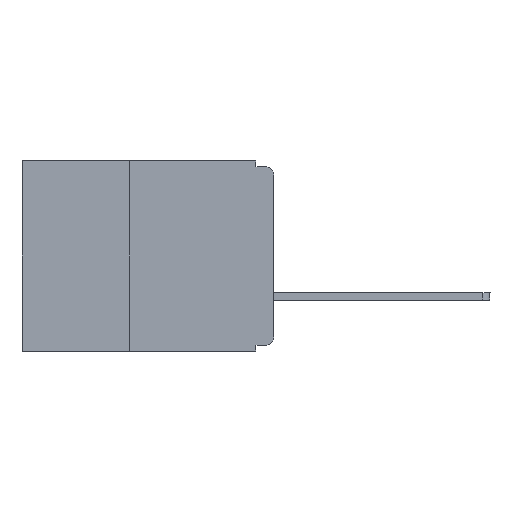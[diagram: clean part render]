
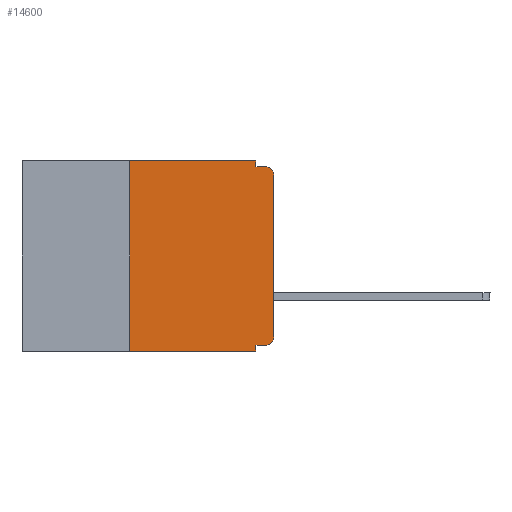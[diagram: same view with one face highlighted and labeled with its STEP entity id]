
A CAD part, left-side view. The second image highlights one B-rep face of the part: STEP entity #14600.
In plain terms, the highlighted planar face has unit normal (-1, 0, 0).
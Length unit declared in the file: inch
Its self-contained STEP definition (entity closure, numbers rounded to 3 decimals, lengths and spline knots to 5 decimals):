
#437 = CARTESIAN_POINT ( 'NONE',  ( 0., 0.031, -0.33 ) ) ;
#593 = EDGE_CURVE ( 'NONE', #3784, #11376, #13927, .T. ) ;
#674 = DIRECTION ( 'NONE',  ( 0., -1., 0. ) ) ;
#755 = EDGE_CURVE ( 'NONE', #5488, #9046, #11928, .T. ) ;
#1028 = EDGE_LOOP ( 'NONE', ( #12949, #4348, #3346, #12899, #10187, #9435, #3592, #7620, #9362, #3938 ) ) ;
#1318 = PLANE ( 'NONE',  #4937 ) ;
#1888 = EDGE_CURVE ( 'NONE', #10842, #5768, #3207, .T. ) ;
#1976 = DIRECTION ( 'NONE',  ( 0., 0., -1. ) ) ;
#2416 = DIRECTION ( 'NONE',  ( 0., 0., -1. ) ) ;
#2444 = CARTESIAN_POINT ( 'NONE',  ( 0., 0.25, -0.33 ) ) ;
#2568 = VERTEX_POINT ( 'NONE', #2605 ) ;
#2590 = EDGE_CURVE ( 'NONE', #4362, #2568, #11555, .T. ) ;
#2605 = CARTESIAN_POINT ( 'NONE',  ( 0., 0.015, -0.01 ) ) ;
#2658 = DIRECTION ( 'NONE',  ( 0., -1., 0. ) ) ;
#2751 = CARTESIAN_POINT ( 'NONE',  ( 0., 0.437, -0.33 ) ) ;
#2938 = DIRECTION ( 'NONE',  ( -1., 0., 0. ) ) ;
#3207 = LINE ( 'NONE', #3568, #4073 ) ;
#3214 = CARTESIAN_POINT ( 'NONE',  ( 0., 0., -0.32 ) ) ;
#3346 = ORIENTED_EDGE ( 'NONE', *, *, #2590, .F. ) ;
#3526 = CARTESIAN_POINT ( 'NONE',  ( 0., 0.031, 0. ) ) ;
#3568 = CARTESIAN_POINT ( 'NONE',  ( 0., 0.437, 0. ) ) ;
#3592 = ORIENTED_EDGE ( 'NONE', *, *, #755, .T. ) ;
#3665 = EDGE_CURVE ( 'NONE', #13156, #2568, #6785, .T. ) ;
#3784 = VERTEX_POINT ( 'NONE', #12173 ) ;
#3938 = ORIENTED_EDGE ( 'NONE', *, *, #10865, .T. ) ;
#4070 = DIRECTION ( 'NONE',  ( 0., 0., -1. ) ) ;
#4073 = VECTOR ( 'NONE', #10389, 39.37008 ) ;
#4074 = CARTESIAN_POINT ( 'NONE',  ( 0., 0.031, 0. ) ) ;
#4137 = CARTESIAN_POINT ( 'NONE',  ( 0., 0.25, 0. ) ) ;
#4348 = ORIENTED_EDGE ( 'NONE', *, *, #3665, .T. ) ;
#4362 = VERTEX_POINT ( 'NONE', #8586 ) ;
#4937 = AXIS2_PLACEMENT_3D ( 'NONE', #6957, #5796, #2416 ) ;
#5096 = DIRECTION ( 'NONE',  ( 0., 0., -1. ) ) ;
#5237 = LINE ( 'NONE', #9715, #11269 ) ;
#5344 = CARTESIAN_POINT ( 'NONE',  ( 0., 0.015, -0.025 ) ) ;
#5423 = CARTESIAN_POINT ( 'NONE',  ( 0., 0., -0.305 ) ) ;
#5488 = VERTEX_POINT ( 'NONE', #13021 ) ;
#5768 = VERTEX_POINT ( 'NONE', #4074 ) ;
#5796 = DIRECTION ( 'NONE',  ( 1., 0., 0. ) ) ;
#6043 = VECTOR ( 'NONE', #9986, 39.37008 ) ;
#6785 = CIRCLE ( 'NONE', #8188, 0.015 ) ;
#6803 = DIRECTION ( 'NONE',  ( 0., 1., 0. ) ) ;
#6957 = CARTESIAN_POINT ( 'NONE',  ( 0., 0.437, 0. ) ) ;
#6969 = VECTOR ( 'NONE', #674, 39.37008 ) ;
#7620 = ORIENTED_EDGE ( 'NONE', *, *, #12825, .F. ) ;
#7634 = CARTESIAN_POINT ( 'NONE',  ( 0., 0., 0. ) ) ;
#7683 = CARTESIAN_POINT ( 'NONE',  ( 0., 0.015, -0.305 ) ) ;
#8010 = LINE ( 'NONE', #2444, #10213 ) ;
#8188 = AXIS2_PLACEMENT_3D ( 'NONE', #5344, #2938, #4070 ) ;
#8586 = CARTESIAN_POINT ( 'NONE',  ( 0., 0.031, -0.01 ) ) ;
#8648 = AXIS2_PLACEMENT_3D ( 'NONE', #7683, #11230, #1976 ) ;
#9046 = VERTEX_POINT ( 'NONE', #437 ) ;
#9179 = CARTESIAN_POINT ( 'NONE',  ( 0., 0.031, -0.32 ) ) ;
#9362 = ORIENTED_EDGE ( 'NONE', *, *, #593, .F. ) ;
#9435 = ORIENTED_EDGE ( 'NONE', *, *, #11553, .F. ) ;
#9715 = CARTESIAN_POINT ( 'NONE',  ( 0., 0.031, -0.33 ) ) ;
#9986 = DIRECTION ( 'NONE',  ( 0., 0., 1. ) ) ;
#10021 = EDGE_CURVE ( 'NONE', #10391, #13156, #10026, .T. ) ;
#10026 = LINE ( 'NONE', #7634, #6043 ) ;
#10187 = ORIENTED_EDGE ( 'NONE', *, *, #1888, .F. ) ;
#10212 = FACE_OUTER_BOUND ( 'NONE', #1028, .T. ) ;
#10213 = VECTOR ( 'NONE', #11744, 39.37008 ) ;
#10389 = DIRECTION ( 'NONE',  ( 0., -1., 0. ) ) ;
#10391 = VERTEX_POINT ( 'NONE', #5423 ) ;
#10485 = CARTESIAN_POINT ( 'NONE',  ( 0., 0., -0.025 ) ) ;
#10842 = VERTEX_POINT ( 'NONE', #4137 ) ;
#10865 = EDGE_CURVE ( 'NONE', #3784, #10391, #14982, .T. ) ;
#11230 = DIRECTION ( 'NONE',  ( -1., 0., 0. ) ) ;
#11269 = VECTOR ( 'NONE', #5096, 39.37008 ) ;
#11376 = VERTEX_POINT ( 'NONE', #9179 ) ;
#11553 = EDGE_CURVE ( 'NONE', #5488, #10842, #8010, .T. ) ;
#11555 = LINE ( 'NONE', #12205, #6969 ) ;
#11678 = DIRECTION ( 'NONE',  ( 0., 0., -1. ) ) ;
#11744 = DIRECTION ( 'NONE',  ( 0., 0., 1. ) ) ;
#11928 = LINE ( 'NONE', #2751, #14846 ) ;
#12173 = CARTESIAN_POINT ( 'NONE',  ( 0., 0.015, -0.32 ) ) ;
#12177 = VECTOR ( 'NONE', #11678, 39.37008 ) ;
#12205 = CARTESIAN_POINT ( 'NONE',  ( 0., 0., -0.01 ) ) ;
#12825 = EDGE_CURVE ( 'NONE', #11376, #9046, #5237, .T. ) ;
#12899 = ORIENTED_EDGE ( 'NONE', *, *, #13137, .F. ) ;
#12949 = ORIENTED_EDGE ( 'NONE', *, *, #10021, .T. ) ;
#13021 = CARTESIAN_POINT ( 'NONE',  ( 0., 0.25, -0.33 ) ) ;
#13137 = EDGE_CURVE ( 'NONE', #5768, #4362, #14919, .T. ) ;
#13156 = VERTEX_POINT ( 'NONE', #10485 ) ;
#13927 = LINE ( 'NONE', #3214, #14283 ) ;
#14283 = VECTOR ( 'NONE', #6803, 39.37008 ) ;
#14600 = ADVANCED_FACE ( 'NONE', ( #10212 ), #1318, .F. ) ;
#14846 = VECTOR ( 'NONE', #2658, 39.37008 ) ;
#14919 = LINE ( 'NONE', #3526, #12177 ) ;
#14982 = CIRCLE ( 'NONE', #8648, 0.015 ) ;
